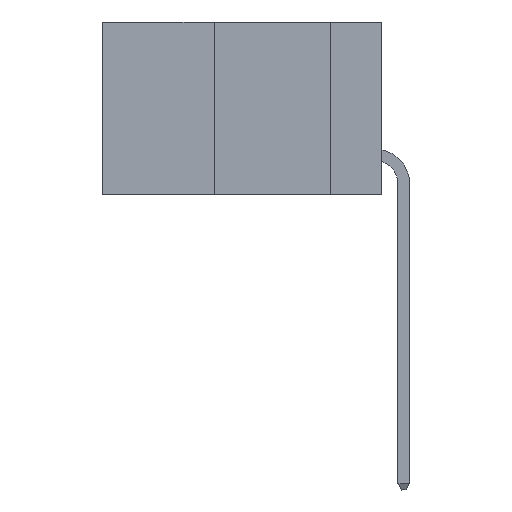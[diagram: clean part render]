
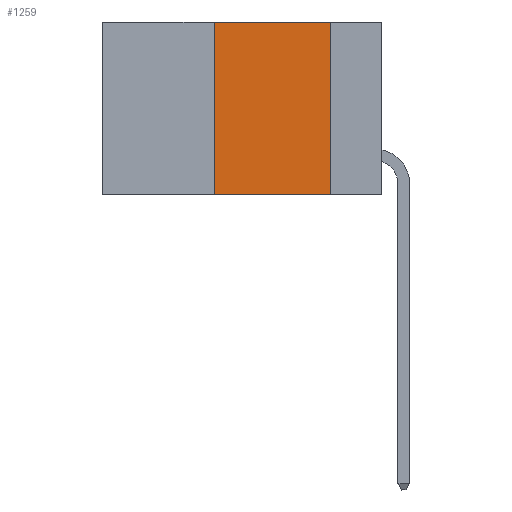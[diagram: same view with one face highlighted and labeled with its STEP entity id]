
A CAD part, left-side view. The second image highlights one B-rep face of the part: STEP entity #1259.
In plain terms, the highlighted planar face has unit normal (-1, 0, 0).
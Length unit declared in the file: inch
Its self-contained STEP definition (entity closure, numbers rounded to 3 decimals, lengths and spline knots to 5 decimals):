
#669 = EDGE_CURVE ( 'NONE', #31507, #20034, #29197, .T. ) ;
#1259 = ADVANCED_FACE ( 'NONE', ( #15911 ), #7669, .F. ) ;
#1475 = LINE ( 'NONE', #6800, #9944 ) ;
#1887 = EDGE_CURVE ( 'NONE', #31507, #17554, #1475, .T. ) ;
#3119 = DIRECTION ( 'NONE',  ( 0., 0., -1. ) ) ;
#4833 = ORIENTED_EDGE ( 'NONE', *, *, #8679, .F. ) ;
#6800 = CARTESIAN_POINT ( 'NONE',  ( 0., 0.36, 0. ) ) ;
#7669 = PLANE ( 'NONE',  #32868 ) ;
#8264 = CARTESIAN_POINT ( 'NONE',  ( 0., 0.11, -0.37 ) ) ;
#8679 = EDGE_CURVE ( 'NONE', #17554, #47860, #41353, .T. ) ;
#9944 = VECTOR ( 'NONE', #21728, 39.37008 ) ;
#10276 = VECTOR ( 'NONE', #3119, 39.37008 ) ;
#11263 = DIRECTION ( 'NONE',  ( 0., -1., 0. ) ) ;
#12775 = DIRECTION ( 'NONE',  ( 0., -1., 0. ) ) ;
#15911 = FACE_OUTER_BOUND ( 'NONE', #38817, .T. ) ;
#16004 = DIRECTION ( 'NONE',  ( 0., 0., -1. ) ) ;
#16093 = CARTESIAN_POINT ( 'NONE',  ( 0., 0.6, -0.37 ) ) ;
#16227 = ORIENTED_EDGE ( 'NONE', *, *, #669, .T. ) ;
#17554 = VERTEX_POINT ( 'NONE', #25573 ) ;
#19334 = CARTESIAN_POINT ( 'NONE',  ( 0., 0.6, 0. ) ) ;
#20034 = VERTEX_POINT ( 'NONE', #8264 ) ;
#20757 = CARTESIAN_POINT ( 'NONE',  ( 0., 0.11, 0. ) ) ;
#21728 = DIRECTION ( 'NONE',  ( 0., 0., 1. ) ) ;
#24286 = CARTESIAN_POINT ( 'NONE',  ( 0., 0.11, 0. ) ) ;
#25573 = CARTESIAN_POINT ( 'NONE',  ( 0., 0.36, 0. ) ) ;
#28065 = LINE ( 'NONE', #24286, #10276 ) ;
#29103 = CARTESIAN_POINT ( 'NONE',  ( 0., 0.36, -0.37 ) ) ;
#29197 = LINE ( 'NONE', #16093, #48057 ) ;
#31353 = DIRECTION ( 'NONE',  ( 1., 0., 0. ) ) ;
#31507 = VERTEX_POINT ( 'NONE', #29103 ) ;
#32868 = AXIS2_PLACEMENT_3D ( 'NONE', #41781, #31353, #16004 ) ;
#34984 = EDGE_CURVE ( 'NONE', #47860, #20034, #28065, .T. ) ;
#35227 = ORIENTED_EDGE ( 'NONE', *, *, #34984, .F. ) ;
#36126 = ORIENTED_EDGE ( 'NONE', *, *, #1887, .F. ) ;
#38817 = EDGE_LOOP ( 'NONE', ( #35227, #4833, #36126, #16227 ) ) ;
#41353 = LINE ( 'NONE', #19334, #41870 ) ;
#41781 = CARTESIAN_POINT ( 'NONE',  ( 0., 0.6, 0. ) ) ;
#41870 = VECTOR ( 'NONE', #11263, 39.37008 ) ;
#47860 = VERTEX_POINT ( 'NONE', #20757 ) ;
#48057 = VECTOR ( 'NONE', #12775, 39.37008 ) ;
